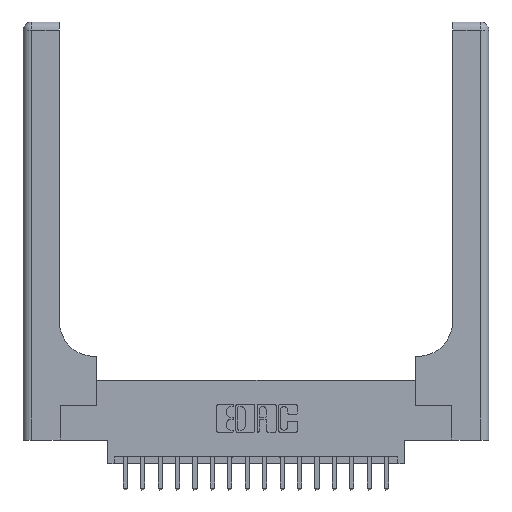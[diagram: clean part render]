
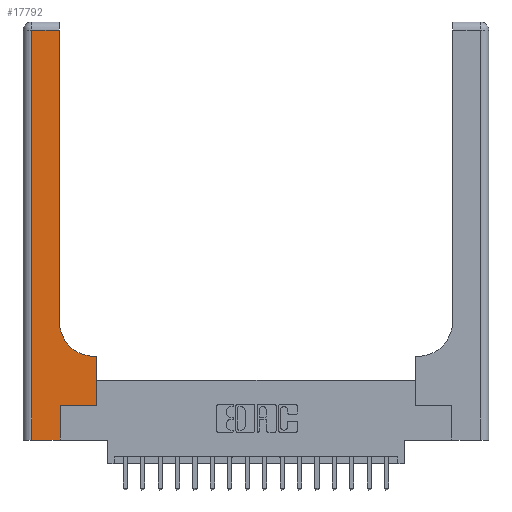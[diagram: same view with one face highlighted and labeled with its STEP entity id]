
A CAD part, top view. The second image highlights one B-rep face of the part: STEP entity #17792.
In plain terms, the highlighted planar face has unit normal (0, 0, 1).
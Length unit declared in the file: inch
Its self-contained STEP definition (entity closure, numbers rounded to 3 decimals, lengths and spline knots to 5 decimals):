
#298 = LINE ( 'NONE', #8871, #7991 ) ;
#590 = LINE ( 'NONE', #10454, #8306 ) ;
#1093 = EDGE_CURVE ( 'NONE', #4608, #18353, #5057, .T. ) ;
#1640 = LINE ( 'NONE', #12033, #9346 ) ;
#1761 = CARTESIAN_POINT ( 'NONE',  ( 0.26, 0.85, 0.37 ) ) ;
#1971 = CARTESIAN_POINT ( 'NONE',  ( 0.26, 0.6, 0.37 ) ) ;
#2034 = LINE ( 'NONE', #2860, #13776 ) ;
#2155 = DIRECTION ( 'NONE',  ( 0., 1., 0. ) ) ;
#2319 = EDGE_CURVE ( 'NONE', #3969, #13725, #1640, .T. ) ;
#2322 = DIRECTION ( 'NONE',  ( 1., 0., 0. ) ) ;
#2343 = DIRECTION ( 'NONE',  ( 0., 0., -1. ) ) ;
#2364 = CARTESIAN_POINT ( 'NONE',  ( 0.51, 0.85, 0.37 ) ) ;
#2860 = CARTESIAN_POINT ( 'NONE',  ( 0.26, 3., 0.37 ) ) ;
#2983 = CARTESIAN_POINT ( 'NONE',  ( 0.265, 0.25, 0.37 ) ) ;
#3085 = VECTOR ( 'NONE', #9752, 39.37008 ) ;
#3509 = DIRECTION ( 'NONE',  ( -1., 0., 0. ) ) ;
#3583 = PLANE ( 'NONE',  #12028 ) ;
#3969 = VERTEX_POINT ( 'NONE', #9607 ) ;
#4221 = DIRECTION ( 'NONE',  ( 1., 0., 0. ) ) ;
#4608 = VERTEX_POINT ( 'NONE', #12885 ) ;
#5028 = VERTEX_POINT ( 'NONE', #8482 ) ;
#5057 = CIRCLE ( 'NONE', #6862, 0.25 ) ;
#5149 = CARTESIAN_POINT ( 'NONE',  ( 0., 3., 0.37 ) ) ;
#5444 = LINE ( 'NONE', #1971, #9064 ) ;
#5529 = EDGE_CURVE ( 'NONE', #18353, #13487, #2034, .T. ) ;
#6603 = ORIENTED_EDGE ( 'NONE', *, *, #5529, .T. ) ;
#6621 = ORIENTED_EDGE ( 'NONE', *, *, #11069, .T. ) ;
#6669 = DIRECTION ( 'NONE',  ( 0., 0., -1. ) ) ;
#6672 = ORIENTED_EDGE ( 'NONE', *, *, #14785, .T. ) ;
#6795 = ORIENTED_EDGE ( 'NONE', *, *, #19054, .T. ) ;
#6815 = ORIENTED_EDGE ( 'NONE', *, *, #2319, .T. ) ;
#6862 = AXIS2_PLACEMENT_3D ( 'NONE', #2364, #2343, #2322 ) ;
#7018 = ORIENTED_EDGE ( 'NONE', *, *, #16982, .T. ) ;
#7026 = LINE ( 'NONE', #8473, #11174 ) ;
#7121 = ORIENTED_EDGE ( 'NONE', *, *, #15983, .T. ) ;
#7161 = ORIENTED_EDGE ( 'NONE', *, *, #13970, .T. ) ;
#7173 = LINE ( 'NONE', #17111, #3085 ) ;
#7259 = ORIENTED_EDGE ( 'NONE', *, *, #1093, .T. ) ;
#7663 = VERTEX_POINT ( 'NONE', #16647 ) ;
#7991 = VECTOR ( 'NONE', #4221, 39.37008 ) ;
#8306 = VECTOR ( 'NONE', #11970, 39.37008 ) ;
#8455 = CARTESIAN_POINT ( 'NONE',  ( 0.26, 2.94, 0.37 ) ) ;
#8473 = CARTESIAN_POINT ( 'NONE',  ( 0., 2.94, 0.37 ) ) ;
#8482 = CARTESIAN_POINT ( 'NONE',  ( 0.528, 0.6, 0.37 ) ) ;
#8871 = CARTESIAN_POINT ( 'NONE',  ( 0.265, 0.25, 0.37 ) ) ;
#9064 = VECTOR ( 'NONE', #3509, 39.37008 ) ;
#9346 = VECTOR ( 'NONE', #11972, 39.37008 ) ;
#9607 = CARTESIAN_POINT ( 'NONE',  ( 0.265, 0., 0.37 ) ) ;
#9752 = DIRECTION ( 'NONE',  ( 1., 0., 0. ) ) ;
#10454 = CARTESIAN_POINT ( 'NONE',  ( 0.06, 3., 0.37 ) ) ;
#10690 = LINE ( 'NONE', #16772, #17991 ) ;
#11069 = EDGE_CURVE ( 'NONE', #13487, #11924, #7026, .T. ) ;
#11092 = EDGE_LOOP ( 'NONE', ( #6603, #6621, #6672, #6795, #6815, #7018, #7121, #7161, #7259 ) ) ;
#11174 = VECTOR ( 'NONE', #18787, 39.37008 ) ;
#11924 = VERTEX_POINT ( 'NONE', #11940 ) ;
#11940 = CARTESIAN_POINT ( 'NONE',  ( 0.06, 2.94, 0.37 ) ) ;
#11970 = DIRECTION ( 'NONE',  ( 0., -1., 0. ) ) ;
#11972 = DIRECTION ( 'NONE',  ( 0., 1., 0. ) ) ;
#12028 = AXIS2_PLACEMENT_3D ( 'NONE', #5149, #6669, #17148 ) ;
#12033 = CARTESIAN_POINT ( 'NONE',  ( 0.265, 0., 0.37 ) ) ;
#12885 = CARTESIAN_POINT ( 'NONE',  ( 0.51, 0.6, 0.37 ) ) ;
#13462 = FACE_OUTER_BOUND ( 'NONE', #11092, .T. ) ;
#13487 = VERTEX_POINT ( 'NONE', #8455 ) ;
#13563 = CARTESIAN_POINT ( 'NONE',  ( 0.528, 0.25, 0.37 ) ) ;
#13725 = VERTEX_POINT ( 'NONE', #2983 ) ;
#13776 = VECTOR ( 'NONE', #2155, 39.37008 ) ;
#13941 = DIRECTION ( 'NONE',  ( 0., 1., 0. ) ) ;
#13970 = EDGE_CURVE ( 'NONE', #5028, #4608, #5444, .T. ) ;
#14785 = EDGE_CURVE ( 'NONE', #11924, #7663, #590, .T. ) ;
#15983 = EDGE_CURVE ( 'NONE', #18146, #5028, #10690, .T. ) ;
#16647 = CARTESIAN_POINT ( 'NONE',  ( 0.06, 0., 0.37 ) ) ;
#16772 = CARTESIAN_POINT ( 'NONE',  ( 0.528, 0.25, 0.37 ) ) ;
#16982 = EDGE_CURVE ( 'NONE', #13725, #18146, #298, .T. ) ;
#17111 = CARTESIAN_POINT ( 'NONE',  ( 0., 0., 0.37 ) ) ;
#17148 = DIRECTION ( 'NONE',  ( -1., 0., 0. ) ) ;
#17792 = ADVANCED_FACE ( 'NONE', ( #13462 ), #3583, .F. ) ;
#17991 = VECTOR ( 'NONE', #13941, 39.37008 ) ;
#18146 = VERTEX_POINT ( 'NONE', #13563 ) ;
#18353 = VERTEX_POINT ( 'NONE', #1761 ) ;
#18787 = DIRECTION ( 'NONE',  ( -1., 0., 0. ) ) ;
#19054 = EDGE_CURVE ( 'NONE', #7663, #3969, #7173, .T. ) ;
